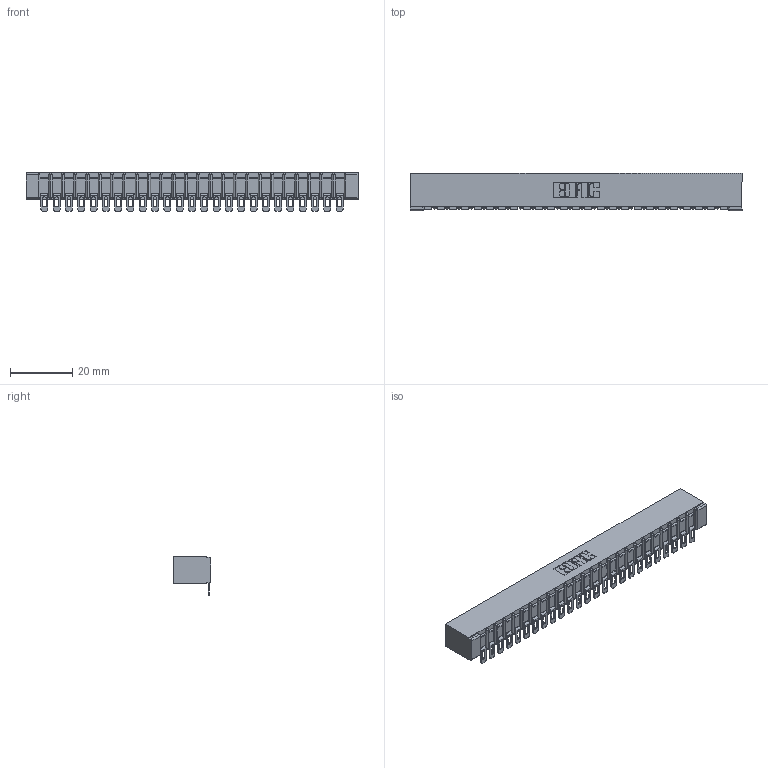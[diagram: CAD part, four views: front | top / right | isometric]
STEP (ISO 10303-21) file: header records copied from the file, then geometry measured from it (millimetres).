
FILE_DESCRIPTION (( 'STEP AP203' ), '1' );
FILE_NAME ('307-025-554-101.STEP', '2018-08-04T13:17:05', ( '' ), ( '' ), 'SwSTEP 2.0', 'SolidWorks 2016', '' );
FILE_SCHEMA (( 'CONFIG_CONTROL_DESIGN' ));
Length unit declared in the file: inch
Products named in the file (3): 307 Part_No Mounting Lugs; 307-290-002_554; 307-025-554-101
Assembly tree (26 placements, depth 2):
  307-025-554-101
    307 Part_No Mounting Lugs
    307-290-002_554  x25
Bounding box: 106.93 x 12.01 x 12.52 mm (x, y, z)
Volume: 7312.5 mm3; surface area: 14077 mm2
Topology: 26 solids, 26 shells, 2161 faces, 6624 edges, 4344 vertices
Faces by surface type: plane 1216, cylinder 893, sphere 52
Entity records: 24215 total; most frequent: CARTESIAN_POINT 4082, ORIENTED_EDGE 4072, DIRECTION 3978, EDGE_CURVE 2036, VECTOR 1546, LINE 1546, VERTEX_POINT 1320, AXIS2_PLACEMENT_3D 1216
